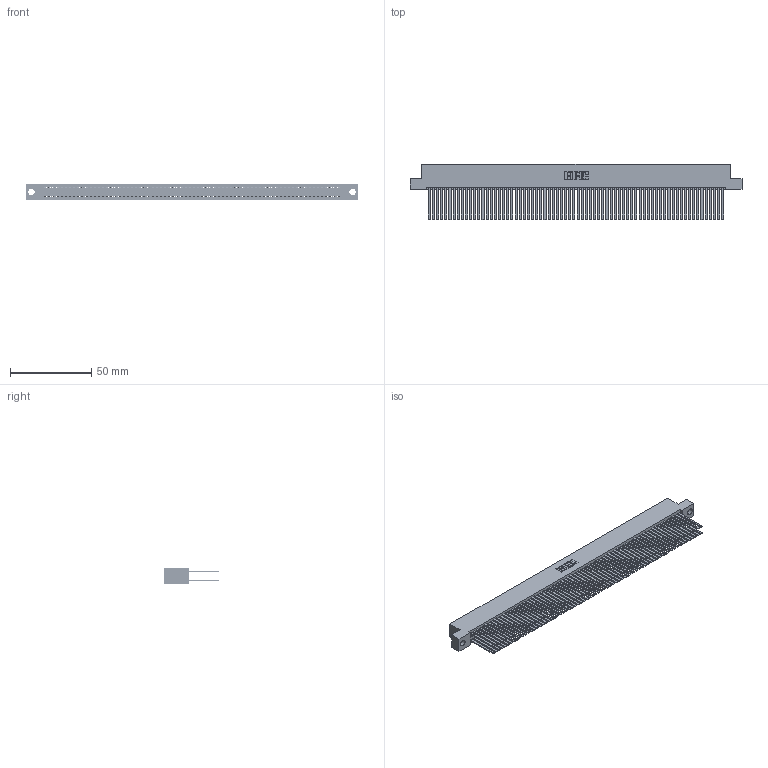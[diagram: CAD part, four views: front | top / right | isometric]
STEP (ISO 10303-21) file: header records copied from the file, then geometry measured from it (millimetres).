
FILE_DESCRIPTION (( 'STEP AP203' ), '1' );
FILE_NAME ('395-144-544-204.STEP', '2018-12-06T09:03:13', ( '' ), ( '' ), 'SwSTEP 2.0', 'SolidWorks 2016', '' );
FILE_SCHEMA (( 'CONFIG_CONTROL_DESIGN' ));
Length unit declared in the file: inch
Products named in the file (3): 395-144-544-204; 345-292-001_345-293-144; 345 Part_Flush Mounting Lugs - 0.156 Dia-TH
Assembly tree (145 placements, depth 2):
  395-144-544-204
    345 Part_Flush Mounting Lugs - 0.156 Dia-TH
    345-292-001_345-293-144  x144
Bounding box: 204.09 x 33.96 x 9.4 mm (x, y, z)
Volume: 22034.6 mm3; surface area: 38883.5 mm2
Topology: 145 solids, 145 shells, 6462 faces, 19205 edges, 12610 vertices
Faces by surface type: plane 4256, cylinder 2206
Entity records: 52273 total; most frequent: CARTESIAN_POINT 8732, ORIENTED_EDGE 8666, DIRECTION 7661, EDGE_CURVE 4333, VECTOR 3917, LINE 3917, VERTEX_POINT 2886, AXIS2_PLACEMENT_3D 1872
